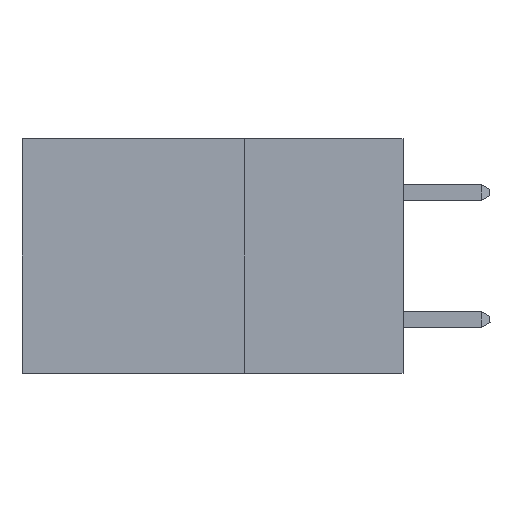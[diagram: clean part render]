
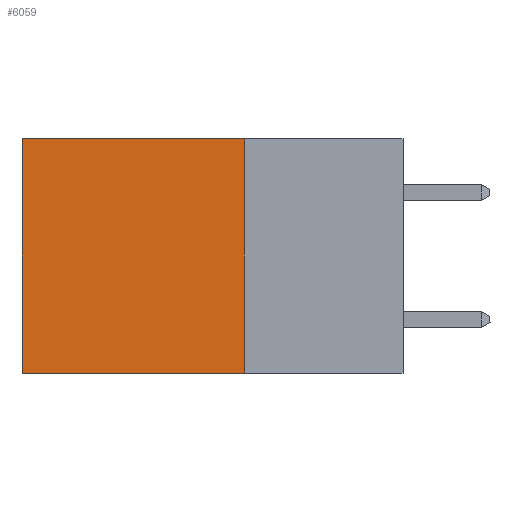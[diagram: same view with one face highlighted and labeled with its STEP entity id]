
A CAD part, left-side view. The second image highlights one B-rep face of the part: STEP entity #6059.
In plain terms, the highlighted planar face has unit normal (-1, 0, 0).
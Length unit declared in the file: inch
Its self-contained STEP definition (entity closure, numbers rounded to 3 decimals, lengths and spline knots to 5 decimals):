
#555 = VECTOR ( 'NONE', #1346, 39.37008 ) ;
#612 = CARTESIAN_POINT ( 'NONE',  ( 0.2875, 0.25, 0. ) ) ;
#737 = EDGE_CURVE ( 'NONE', #16105, #8387, #19037, .T. ) ;
#1022 = FACE_OUTER_BOUND ( 'NONE', #10104, .T. ) ;
#1346 = DIRECTION ( 'NONE',  ( 0., 1., 0. ) ) ;
#1499 = AXIS2_PLACEMENT_3D ( 'NONE', #8084, #23885, #10406 ) ;
#3017 = DIRECTION ( 'NONE',  ( 0., 0., -1. ) ) ;
#3281 = ORIENTED_EDGE ( 'NONE', *, *, #24548, .F. ) ;
#3490 = ORIENTED_EDGE ( 'NONE', *, *, #737, .F. ) ;
#4279 = LINE ( 'NONE', #6158, #27762 ) ;
#5203 = EDGE_CURVE ( 'NONE', #13037, #18407, #18108, .T. ) ;
#6059 = ADVANCED_FACE ( 'NONE', ( #1022 ), #21657, .F. ) ;
#6158 = CARTESIAN_POINT ( 'NONE',  ( 0.2875, 0.6, 0. ) ) ;
#6627 = ORIENTED_EDGE ( 'NONE', *, *, #17500, .T. ) ;
#6801 = CARTESIAN_POINT ( 'NONE',  ( 0.2875, 0.6, -0.37 ) ) ;
#8084 = CARTESIAN_POINT ( 'NONE',  ( 0.2875, 0.25, 0. ) ) ;
#8387 = VERTEX_POINT ( 'NONE', #6801 ) ;
#8676 = ORIENTED_EDGE ( 'NONE', *, *, #5203, .T. ) ;
#10104 = EDGE_LOOP ( 'NONE', ( #6627, #3490, #3281, #8676 ) ) ;
#10406 = DIRECTION ( 'NONE',  ( 0., 0., -1. ) ) ;
#10742 = CARTESIAN_POINT ( 'NONE',  ( 0.2875, 0.25, -0.37 ) ) ;
#10867 = CARTESIAN_POINT ( 'NONE',  ( 0.2875, 0.25, 0. ) ) ;
#10893 = DIRECTION ( 'NONE',  ( 0., 0., -1. ) ) ;
#12125 = VECTOR ( 'NONE', #21354, 39.37008 ) ;
#12323 = CARTESIAN_POINT ( 'NONE',  ( 0.2875, 0.25, 0. ) ) ;
#13037 = VERTEX_POINT ( 'NONE', #10867 ) ;
#15666 = VECTOR ( 'NONE', #3017, 39.37008 ) ;
#15982 = CARTESIAN_POINT ( 'NONE',  ( 0.2875, 0.6, 0. ) ) ;
#16105 = VERTEX_POINT ( 'NONE', #17379 ) ;
#17379 = CARTESIAN_POINT ( 'NONE',  ( 0.2875, 0.25, -0.37 ) ) ;
#17500 = EDGE_CURVE ( 'NONE', #18407, #8387, #4279, .T. ) ;
#18108 = LINE ( 'NONE', #12323, #12125 ) ;
#18407 = VERTEX_POINT ( 'NONE', #15982 ) ;
#19037 = LINE ( 'NONE', #10742, #555 ) ;
#21354 = DIRECTION ( 'NONE',  ( 0., 1., 0. ) ) ;
#21657 = PLANE ( 'NONE',  #1499 ) ;
#23043 = LINE ( 'NONE', #612, #15666 ) ;
#23885 = DIRECTION ( 'NONE',  ( 1., 0., 0. ) ) ;
#24548 = EDGE_CURVE ( 'NONE', #13037, #16105, #23043, .T. ) ;
#27762 = VECTOR ( 'NONE', #10893, 39.37008 ) ;
